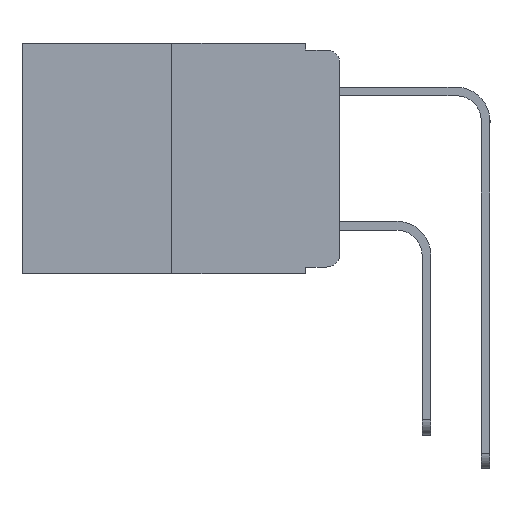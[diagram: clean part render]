
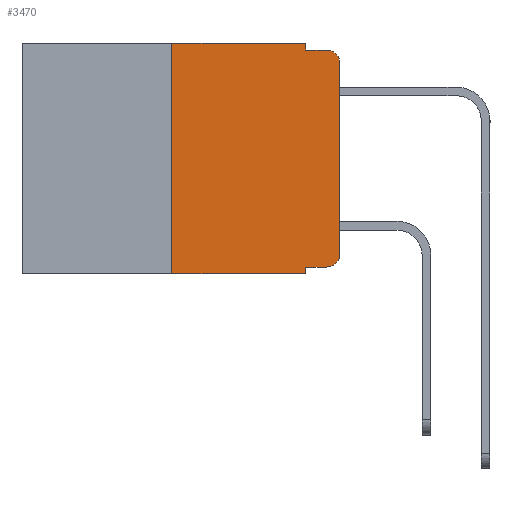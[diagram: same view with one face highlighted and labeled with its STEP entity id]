
A CAD part, left-side view. The second image highlights one B-rep face of the part: STEP entity #3470.
In plain terms, the highlighted planar face has unit normal (-1, 0, 0).
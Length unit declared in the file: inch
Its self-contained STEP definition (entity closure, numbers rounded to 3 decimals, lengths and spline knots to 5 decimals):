
#108 = ORIENTED_EDGE ( 'NONE', *, *, #15649, .T. ) ;
#130 = VERTEX_POINT ( 'NONE', #16635 ) ;
#154 = CARTESIAN_POINT ( 'NONE',  ( 0., 0.473, 0. ) ) ;
#1206 = DIRECTION ( 'NONE',  ( 0., 0., -1. ) ) ;
#1369 = LINE ( 'NONE', #5116, #8206 ) ;
#1594 = ORIENTED_EDGE ( 'NONE', *, *, #4271, .T. ) ;
#1772 = EDGE_CURVE ( 'NONE', #2394, #4602, #1369, .T. ) ;
#2394 = VERTEX_POINT ( 'NONE', #10218 ) ;
#3002 = ORIENTED_EDGE ( 'NONE', *, *, #3246, .F. ) ;
#3176 = VERTEX_POINT ( 'NONE', #13878 ) ;
#3246 = EDGE_CURVE ( 'NONE', #15544, #130, #9795, .T. ) ;
#3264 = LINE ( 'NONE', #12653, #13281 ) ;
#3298 = FACE_OUTER_BOUND ( 'NONE', #6381, .T. ) ;
#3470 = ADVANCED_FACE ( 'NONE', ( #3298 ), #6640, .F. ) ;
#3638 = CARTESIAN_POINT ( 'NONE',  ( 0., 0.25, 0. ) ) ;
#3743 = DIRECTION ( 'NONE',  ( 0., 0., -1. ) ) ;
#4049 = ORIENTED_EDGE ( 'NONE', *, *, #1772, .F. ) ;
#4271 = EDGE_CURVE ( 'NONE', #7010, #16410, #15988, .T. ) ;
#4418 = ORIENTED_EDGE ( 'NONE', *, *, #5233, .F. ) ;
#4421 = EDGE_CURVE ( 'NONE', #11606, #4602, #3264, .T. ) ;
#4447 = DIRECTION ( 'NONE',  ( 0., -1., 0. ) ) ;
#4602 = VERTEX_POINT ( 'NONE', #8123 ) ;
#4859 = CARTESIAN_POINT ( 'NONE',  ( 0., 0.25, 0. ) ) ;
#5001 = DIRECTION ( 'NONE',  ( 0., 0., -1. ) ) ;
#5116 = CARTESIAN_POINT ( 'NONE',  ( 0., 0.051, 0. ) ) ;
#5233 = EDGE_CURVE ( 'NONE', #130, #11088, #11739, .T. ) ;
#5849 = CARTESIAN_POINT ( 'NONE',  ( 0., 0.02, -0.01 ) ) ;
#6055 = AXIS2_PLACEMENT_3D ( 'NONE', #15387, #14933, #5001 ) ;
#6381 = EDGE_LOOP ( 'NONE', ( #1594, #7578, #13527, #4418, #3002, #6746, #14352, #4049, #6807, #108 ) ) ;
#6640 = PLANE ( 'NONE',  #6055 ) ;
#6746 = ORIENTED_EDGE ( 'NONE', *, *, #11058, .F. ) ;
#6807 = ORIENTED_EDGE ( 'NONE', *, *, #12424, .T. ) ;
#6832 = EDGE_CURVE ( 'NONE', #11088, #7667, #16313, .T. ) ;
#6992 = EDGE_CURVE ( 'NONE', #16410, #7667, #14786, .T. ) ;
#7010 = VERTEX_POINT ( 'NONE', #11831 ) ;
#7086 = DIRECTION ( 'NONE',  ( 0., 0., -1. ) ) ;
#7104 = CIRCLE ( 'NONE', #14323, 0.02 ) ;
#7524 = CARTESIAN_POINT ( 'NONE',  ( 0., 0., 0. ) ) ;
#7578 = ORIENTED_EDGE ( 'NONE', *, *, #6992, .T. ) ;
#7667 = VERTEX_POINT ( 'NONE', #5849 ) ;
#7957 = DIRECTION ( 'NONE',  ( 0., -1., 0. ) ) ;
#8123 = CARTESIAN_POINT ( 'NONE',  ( 0., 0.051, -0.343 ) ) ;
#8206 = VECTOR ( 'NONE', #3743, 39.37008 ) ;
#8612 = VECTOR ( 'NONE', #7957, 39.37008 ) ;
#9316 = DIRECTION ( 'NONE',  ( -1., 0., 0. ) ) ;
#9382 = VECTOR ( 'NONE', #4447, 39.37008 ) ;
#9448 = DIRECTION ( 'NONE',  ( 0., -1., 0. ) ) ;
#9795 = LINE ( 'NONE', #154, #9382 ) ;
#10218 = CARTESIAN_POINT ( 'NONE',  ( 0., 0.051, -0.333 ) ) ;
#11058 = EDGE_CURVE ( 'NONE', #11606, #15544, #15724, .T. ) ;
#11088 = VERTEX_POINT ( 'NONE', #13950 ) ;
#11181 = DIRECTION ( 'NONE',  ( 0., -1., 0. ) ) ;
#11329 = VECTOR ( 'NONE', #7086, 39.37008 ) ;
#11606 = VERTEX_POINT ( 'NONE', #12531 ) ;
#11712 = CARTESIAN_POINT ( 'NONE',  ( 0., 0.051, -0.01 ) ) ;
#11739 = LINE ( 'NONE', #13506, #11329 ) ;
#11831 = CARTESIAN_POINT ( 'NONE',  ( 0., 0., -0.313 ) ) ;
#11962 = AXIS2_PLACEMENT_3D ( 'NONE', #15338, #15264, #15377 ) ;
#12258 = VECTOR ( 'NONE', #11181, 39.37008 ) ;
#12424 = EDGE_CURVE ( 'NONE', #2394, #3176, #14910, .T. ) ;
#12531 = CARTESIAN_POINT ( 'NONE',  ( 0., 0.25, -0.343 ) ) ;
#12653 = CARTESIAN_POINT ( 'NONE',  ( 0., 0.473, -0.343 ) ) ;
#12657 = DIRECTION ( 'NONE',  ( 0., 0., 1. ) ) ;
#12707 = VECTOR ( 'NONE', #14716, 39.37008 ) ;
#12818 = VECTOR ( 'NONE', #12657, 39.37008 ) ;
#13100 = CARTESIAN_POINT ( 'NONE',  ( 0., 0., -0.03 ) ) ;
#13281 = VECTOR ( 'NONE', #9448, 39.37008 ) ;
#13506 = CARTESIAN_POINT ( 'NONE',  ( 0., 0.051, 0. ) ) ;
#13527 = ORIENTED_EDGE ( 'NONE', *, *, #6832, .F. ) ;
#13878 = CARTESIAN_POINT ( 'NONE',  ( 0., 0.02, -0.333 ) ) ;
#13950 = CARTESIAN_POINT ( 'NONE',  ( 0., 0.051, -0.01 ) ) ;
#14323 = AXIS2_PLACEMENT_3D ( 'NONE', #16755, #9316, #1206 ) ;
#14352 = ORIENTED_EDGE ( 'NONE', *, *, #4421, .T. ) ;
#14716 = DIRECTION ( 'NONE',  ( 0., 0., 1. ) ) ;
#14786 = CIRCLE ( 'NONE', #11962, 0.02 ) ;
#14910 = LINE ( 'NONE', #15471, #8612 ) ;
#14933 = DIRECTION ( 'NONE',  ( 1., 0., 0. ) ) ;
#15264 = DIRECTION ( 'NONE',  ( -1., 0., 0. ) ) ;
#15338 = CARTESIAN_POINT ( 'NONE',  ( 0., 0.02, -0.03 ) ) ;
#15377 = DIRECTION ( 'NONE',  ( 0., 0., -1. ) ) ;
#15387 = CARTESIAN_POINT ( 'NONE',  ( 0., 0.473, 0. ) ) ;
#15471 = CARTESIAN_POINT ( 'NONE',  ( 0., 0.051, -0.333 ) ) ;
#15544 = VERTEX_POINT ( 'NONE', #3638 ) ;
#15649 = EDGE_CURVE ( 'NONE', #3176, #7010, #7104, .T. ) ;
#15724 = LINE ( 'NONE', #4859, #12818 ) ;
#15988 = LINE ( 'NONE', #7524, #12707 ) ;
#16313 = LINE ( 'NONE', #11712, #12258 ) ;
#16410 = VERTEX_POINT ( 'NONE', #13100 ) ;
#16635 = CARTESIAN_POINT ( 'NONE',  ( 0., 0.051, 0. ) ) ;
#16755 = CARTESIAN_POINT ( 'NONE',  ( 0., 0.02, -0.313 ) ) ;
